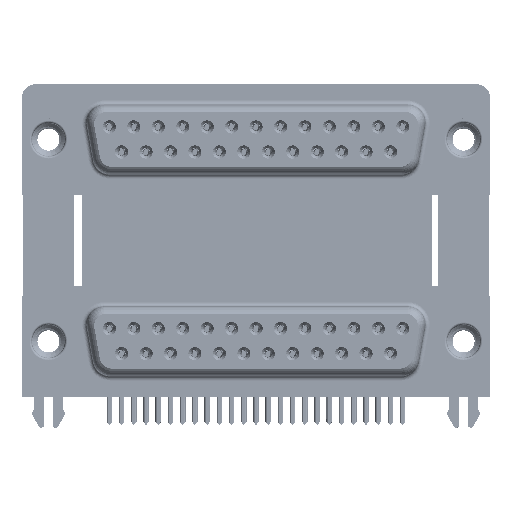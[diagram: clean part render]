
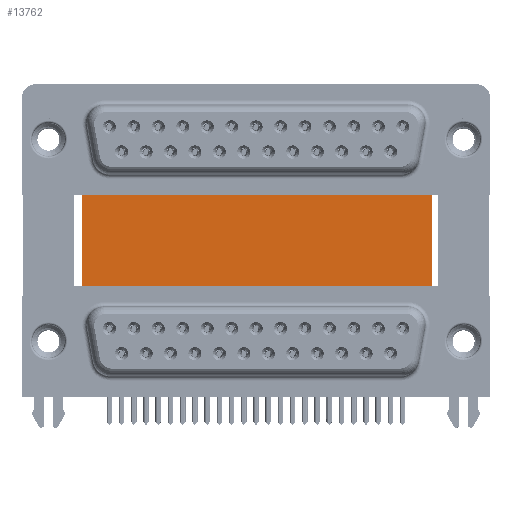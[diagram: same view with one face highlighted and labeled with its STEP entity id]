
A CAD part, top view. The second image highlights one B-rep face of the part: STEP entity #13762.
In plain terms, the highlighted planar face has unit normal (0, 0, 1).
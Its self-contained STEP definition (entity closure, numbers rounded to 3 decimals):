
#74 = ORIENTED_EDGE ( 'NONE', *, *, #39976, .T. ) ;
#2172 = DIRECTION ( 'NONE',  ( -1., 0., 0. ) ) ;
#3237 = DIRECTION ( 'NONE',  ( 0., -1., 0. ) ) ;
#3900 = LINE ( 'NONE', #28790, #49017 ) ;
#8335 = LINE ( 'NONE', #38033, #22008 ) ;
#9366 = DIRECTION ( 'NONE',  ( 1., 0., 0. ) ) ;
#11154 = VERTEX_POINT ( 'NONE', #45687 ) ;
#11657 = LINE ( 'NONE', #12599, #61591 ) ;
#12599 = CARTESIAN_POINT ( 'NONE',  ( 43.43, 16.585, -12. ) ) ;
#13462 = DIRECTION ( 'NONE',  ( 1., 0., 0. ) ) ;
#13762 = ADVANCED_FACE ( 'NONE', ( #26447 ), #25513, .F. ) ;
#18949 = LINE ( 'NONE', #48677, #61659 ) ;
#21963 = DIRECTION ( 'NONE',  ( 0., 0., -1. ) ) ;
#22006 = EDGE_CURVE ( 'NONE', #34248, #35687, #8335, .T. ) ;
#22008 = VECTOR ( 'NONE', #3237, 1000. ) ;
#25513 = PLANE ( 'NONE',  #58842 ) ;
#26447 = FACE_OUTER_BOUND ( 'NONE', #35285, .T. ) ;
#27279 = DIRECTION ( 'NONE',  ( 0., -1., 0. ) ) ;
#28790 = CARTESIAN_POINT ( 'NONE',  ( 3.79, -3.735, -12. ) ) ;
#30032 = EDGE_CURVE ( 'NONE', #34248, #11154, #18949, .T. ) ;
#30936 = CARTESIAN_POINT ( 'NONE',  ( 3.79, 16.585, -12. ) ) ;
#33864 = ORIENTED_EDGE ( 'NONE', *, *, #22006, .T. ) ;
#34248 = VERTEX_POINT ( 'NONE', #38597 ) ;
#35285 = EDGE_LOOP ( 'NONE', ( #74, #36528, #39645, #33864 ) ) ;
#35687 = VERTEX_POINT ( 'NONE', #44587 ) ;
#36528 = ORIENTED_EDGE ( 'NONE', *, *, #47009, .F. ) ;
#38033 = CARTESIAN_POINT ( 'NONE',  ( 3.79, 16.585, -12. ) ) ;
#38597 = CARTESIAN_POINT ( 'NONE',  ( 3.79, 16.585, -12. ) ) ;
#39092 = CARTESIAN_POINT ( 'NONE',  ( 43.43, -3.735, -12. ) ) ;
#39645 = ORIENTED_EDGE ( 'NONE', *, *, #30032, .F. ) ;
#39976 = EDGE_CURVE ( 'NONE', #35687, #52373, #3900, .T. ) ;
#44587 = CARTESIAN_POINT ( 'NONE',  ( 3.79, -3.735, -12. ) ) ;
#45687 = CARTESIAN_POINT ( 'NONE',  ( 43.43, 16.585, -12. ) ) ;
#47009 = EDGE_CURVE ( 'NONE', #11154, #52373, #11657, .T. ) ;
#48677 = CARTESIAN_POINT ( 'NONE',  ( 3.79, 16.585, -12. ) ) ;
#49017 = VECTOR ( 'NONE', #13462, 1000. ) ;
#52373 = VERTEX_POINT ( 'NONE', #39092 ) ;
#58842 = AXIS2_PLACEMENT_3D ( 'NONE', #30936, #21963, #2172 ) ;
#61591 = VECTOR ( 'NONE', #27279, 1000. ) ;
#61659 = VECTOR ( 'NONE', #9366, 1000. ) ;
